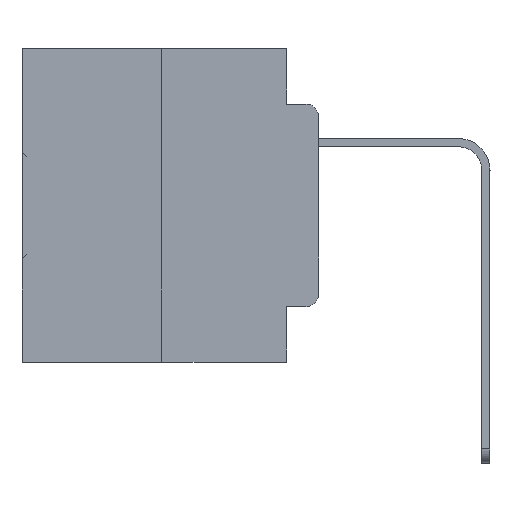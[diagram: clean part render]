
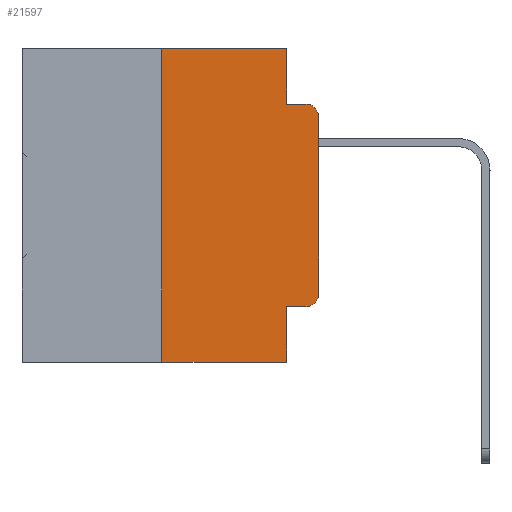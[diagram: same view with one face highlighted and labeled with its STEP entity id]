
A CAD part, left-side view. The second image highlights one B-rep face of the part: STEP entity #21597.
In plain terms, the highlighted planar face has unit normal (-1, 0, 0).
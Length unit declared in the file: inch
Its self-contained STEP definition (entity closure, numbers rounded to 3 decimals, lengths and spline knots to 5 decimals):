
#1305 = EDGE_CURVE ( 'NONE', #20064, #19752, #15266, .T. ) ;
#1618 = ORIENTED_EDGE ( 'NONE', *, *, #30234, .T. ) ;
#1624 = CARTESIAN_POINT ( 'NONE',  ( 0., 0.051, 0. ) ) ;
#1703 = ORIENTED_EDGE ( 'NONE', *, *, #6542, .T. ) ;
#1808 = ORIENTED_EDGE ( 'NONE', *, *, #1305, .F. ) ;
#2657 = DIRECTION ( 'NONE',  ( 0., 0., 1. ) ) ;
#2766 = LINE ( 'NONE', #1624, #20247 ) ;
#2913 = CARTESIAN_POINT ( 'NONE',  ( 0., 0.051, -0.4115 ) ) ;
#3250 = ORIENTED_EDGE ( 'NONE', *, *, #13019, .F. ) ;
#3477 = EDGE_CURVE ( 'NONE', #18121, #4635, #25442, .T. ) ;
#3596 = DIRECTION ( 'NONE',  ( 0., -1., 0. ) ) ;
#4208 = LINE ( 'NONE', #27664, #27986 ) ;
#4635 = VERTEX_POINT ( 'NONE', #17100 ) ;
#5240 = PLANE ( 'NONE',  #32766 ) ;
#5764 = VECTOR ( 'NONE', #32787, 39.37008 ) ;
#6332 = ORIENTED_EDGE ( 'NONE', *, *, #31690, .F. ) ;
#6380 = EDGE_CURVE ( 'NONE', #22509, #11157, #2766, .T. ) ;
#6542 = EDGE_CURVE ( 'NONE', #32812, #11157, #29741, .T. ) ;
#7658 = AXIS2_PLACEMENT_3D ( 'NONE', #24782, #9438, #17207 ) ;
#9438 = DIRECTION ( 'NONE',  ( -1., 0., 0. ) ) ;
#9453 = DIRECTION ( 'NONE',  ( 0., 0., -1. ) ) ;
#9479 = DIRECTION ( 'NONE',  ( 0., 0., -1. ) ) ;
#10678 = EDGE_CURVE ( 'NONE', #22363, #22790, #27312, .T. ) ;
#10967 = CARTESIAN_POINT ( 'NONE',  ( 0., 0.25, 0. ) ) ;
#11103 = CARTESIAN_POINT ( 'NONE',  ( 0., 0.473, 0. ) ) ;
#11157 = VERTEX_POINT ( 'NONE', #13727 ) ;
#11247 = VERTEX_POINT ( 'NONE', #29272 ) ;
#12025 = CARTESIAN_POINT ( 'NONE',  ( 0., 0.02, -0.1085 ) ) ;
#12253 = VECTOR ( 'NONE', #15535, 39.37008 ) ;
#12348 = VECTOR ( 'NONE', #29316, 39.37008 ) ;
#12657 = ORIENTED_EDGE ( 'NONE', *, *, #6380, .F. ) ;
#13019 = EDGE_CURVE ( 'NONE', #32812, #18121, #29112, .T. ) ;
#13065 = CARTESIAN_POINT ( 'NONE',  ( 0., 0.473, 0. ) ) ;
#13485 = VECTOR ( 'NONE', #3596, 39.37008 ) ;
#13727 = CARTESIAN_POINT ( 'NONE',  ( 0., 0.051, -0.5 ) ) ;
#13996 = DIRECTION ( 'NONE',  ( 0., 0., -1. ) ) ;
#14297 = EDGE_CURVE ( 'NONE', #22509, #22363, #21145, .T. ) ;
#14512 = LINE ( 'NONE', #19123, #20083 ) ;
#14661 = CARTESIAN_POINT ( 'NONE',  ( 0., 0.02, -0.4115 ) ) ;
#14999 = DIRECTION ( 'NONE',  ( 0., 0., 1. ) ) ;
#15096 = CARTESIAN_POINT ( 'NONE',  ( 0., 0.473, -0.5 ) ) ;
#15266 = LINE ( 'NONE', #30330, #5764 ) ;
#15535 = DIRECTION ( 'NONE',  ( 0., -1., 0. ) ) ;
#15550 = FACE_OUTER_BOUND ( 'NONE', #17276, .T. ) ;
#15719 = ORIENTED_EDGE ( 'NONE', *, *, #14297, .T. ) ;
#17100 = CARTESIAN_POINT ( 'NONE',  ( 0., 0.051, 0. ) ) ;
#17155 = CIRCLE ( 'NONE', #23137, 0.02 ) ;
#17207 = DIRECTION ( 'NONE',  ( 0., 0., -1. ) ) ;
#17276 = EDGE_LOOP ( 'NONE', ( #18477, #1618, #1808, #6332, #25523, #3250, #1703, #12657, #15719, #29091 ) ) ;
#17414 = CARTESIAN_POINT ( 'NONE',  ( 0., 0.02, -0.0885 ) ) ;
#18121 = VERTEX_POINT ( 'NONE', #31992 ) ;
#18477 = ORIENTED_EDGE ( 'NONE', *, *, #23944, .T. ) ;
#19029 = CARTESIAN_POINT ( 'NONE',  ( 0., 0.051, -0.4115 ) ) ;
#19123 = CARTESIAN_POINT ( 'NONE',  ( 0., 0.051, 0. ) ) ;
#19439 = CARTESIAN_POINT ( 'NONE',  ( 0., 0., -0.3915 ) ) ;
#19752 = VERTEX_POINT ( 'NONE', #17414 ) ;
#19932 = DIRECTION ( 'NONE',  ( -1., 0., 0. ) ) ;
#20064 = VERTEX_POINT ( 'NONE', #26417 ) ;
#20083 = VECTOR ( 'NONE', #13996, 39.37008 ) ;
#20247 = VECTOR ( 'NONE', #9453, 39.37008 ) ;
#21145 = LINE ( 'NONE', #19029, #12348 ) ;
#21502 = CARTESIAN_POINT ( 'NONE',  ( 0., 0.25, -0.5 ) ) ;
#21597 = ADVANCED_FACE ( 'NONE', ( #15550 ), #5240, .F. ) ;
#22363 = VERTEX_POINT ( 'NONE', #14661 ) ;
#22509 = VERTEX_POINT ( 'NONE', #2913 ) ;
#22790 = VERTEX_POINT ( 'NONE', #19439 ) ;
#23137 = AXIS2_PLACEMENT_3D ( 'NONE', #12025, #19932, #9479 ) ;
#23944 = EDGE_CURVE ( 'NONE', #22790, #11247, #4208, .T. ) ;
#24782 = CARTESIAN_POINT ( 'NONE',  ( 0., 0.02, -0.3915 ) ) ;
#25442 = LINE ( 'NONE', #11103, #13485 ) ;
#25523 = ORIENTED_EDGE ( 'NONE', *, *, #3477, .F. ) ;
#26417 = CARTESIAN_POINT ( 'NONE',  ( 0., 0.051, -0.0885 ) ) ;
#27312 = CIRCLE ( 'NONE', #7658, 0.02 ) ;
#27664 = CARTESIAN_POINT ( 'NONE',  ( 0., 0., 0. ) ) ;
#27845 = DIRECTION ( 'NONE',  ( 0., 0., -1. ) ) ;
#27986 = VECTOR ( 'NONE', #14999, 39.37008 ) ;
#29091 = ORIENTED_EDGE ( 'NONE', *, *, #10678, .T. ) ;
#29112 = LINE ( 'NONE', #10967, #29484 ) ;
#29272 = CARTESIAN_POINT ( 'NONE',  ( 0., 0., -0.1085 ) ) ;
#29316 = DIRECTION ( 'NONE',  ( 0., -1., 0. ) ) ;
#29484 = VECTOR ( 'NONE', #2657, 39.37008 ) ;
#29741 = LINE ( 'NONE', #15096, #12253 ) ;
#30234 = EDGE_CURVE ( 'NONE', #11247, #19752, #17155, .T. ) ;
#30330 = CARTESIAN_POINT ( 'NONE',  ( 0., 0.051, -0.0885 ) ) ;
#30839 = DIRECTION ( 'NONE',  ( 1., 0., 0. ) ) ;
#31690 = EDGE_CURVE ( 'NONE', #4635, #20064, #14512, .T. ) ;
#31992 = CARTESIAN_POINT ( 'NONE',  ( 0., 0.25, 0. ) ) ;
#32766 = AXIS2_PLACEMENT_3D ( 'NONE', #13065, #30839, #27845 ) ;
#32787 = DIRECTION ( 'NONE',  ( 0., -1., 0. ) ) ;
#32812 = VERTEX_POINT ( 'NONE', #21502 ) ;
